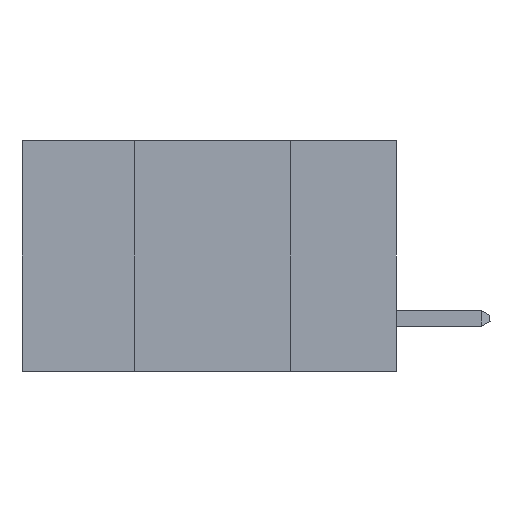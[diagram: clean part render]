
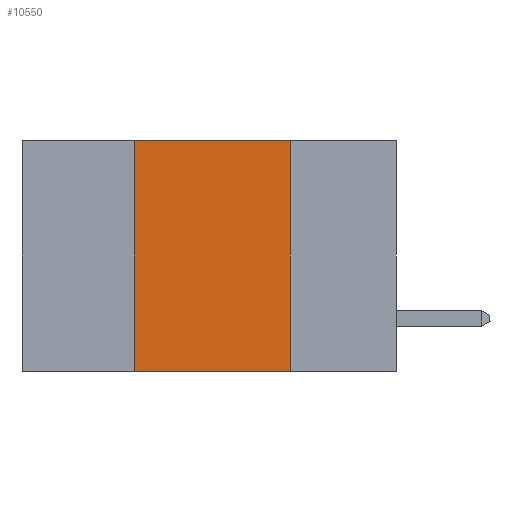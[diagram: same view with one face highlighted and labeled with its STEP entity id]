
A CAD part, left-side view. The second image highlights one B-rep face of the part: STEP entity #10550.
In plain terms, the highlighted planar face has unit normal (-1, 0, 0).
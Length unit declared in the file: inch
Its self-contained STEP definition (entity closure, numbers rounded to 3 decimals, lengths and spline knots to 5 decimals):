
#1699 = CARTESIAN_POINT ( 'NONE',  ( 0., 0.17, 0. ) ) ;
#2723 = DIRECTION ( 'NONE',  ( 0., 0., 1. ) ) ;
#2768 = CARTESIAN_POINT ( 'NONE',  ( 0., 0.17, 0. ) ) ;
#3005 = VERTEX_POINT ( 'NONE', #1699 ) ;
#3600 = EDGE_CURVE ( 'NONE', #3005, #13760, #9320, .T. ) ;
#3969 = CARTESIAN_POINT ( 'NONE',  ( 0., 0.6, -0.37 ) ) ;
#4650 = VERTEX_POINT ( 'NONE', #13246 ) ;
#6016 = VERTEX_POINT ( 'NONE', #13065 ) ;
#6227 = CARTESIAN_POINT ( 'NONE',  ( 0., 0.42, 0. ) ) ;
#6382 = ORIENTED_EDGE ( 'NONE', *, *, #3600, .F. ) ;
#6568 = VECTOR ( 'NONE', #2723, 39.37008 ) ;
#6905 = VECTOR ( 'NONE', #17287, 39.37008 ) ;
#7635 = AXIS2_PLACEMENT_3D ( 'NONE', #21035, #19313, #11101 ) ;
#7870 = EDGE_CURVE ( 'NONE', #4650, #3005, #17829, .T. ) ;
#8924 = CARTESIAN_POINT ( 'NONE',  ( 0., 0.6, 0. ) ) ;
#8963 = ORIENTED_EDGE ( 'NONE', *, *, #17254, .T. ) ;
#9320 = LINE ( 'NONE', #2768, #18553 ) ;
#10550 = ADVANCED_FACE ( 'NONE', ( #16448 ), #17581, .F. ) ;
#11101 = DIRECTION ( 'NONE',  ( 0., 0., -1. ) ) ;
#11475 = LINE ( 'NONE', #6227, #6568 ) ;
#11549 = EDGE_LOOP ( 'NONE', ( #6382, #18554, #17080, #8963 ) ) ;
#13065 = CARTESIAN_POINT ( 'NONE',  ( 0., 0.42, -0.37 ) ) ;
#13144 = VECTOR ( 'NONE', #17275, 39.37008 ) ;
#13246 = CARTESIAN_POINT ( 'NONE',  ( 0., 0.42, 0. ) ) ;
#13629 = LINE ( 'NONE', #3969, #6905 ) ;
#13760 = VERTEX_POINT ( 'NONE', #17978 ) ;
#15643 = EDGE_CURVE ( 'NONE', #6016, #4650, #11475, .T. ) ;
#16448 = FACE_OUTER_BOUND ( 'NONE', #11549, .T. ) ;
#17080 = ORIENTED_EDGE ( 'NONE', *, *, #15643, .F. ) ;
#17254 = EDGE_CURVE ( 'NONE', #6016, #13760, #13629, .T. ) ;
#17275 = DIRECTION ( 'NONE',  ( 0., -1., 0. ) ) ;
#17287 = DIRECTION ( 'NONE',  ( 0., -1., 0. ) ) ;
#17581 = PLANE ( 'NONE',  #7635 ) ;
#17829 = LINE ( 'NONE', #8924, #13144 ) ;
#17978 = CARTESIAN_POINT ( 'NONE',  ( 0., 0.17, -0.37 ) ) ;
#18553 = VECTOR ( 'NONE', #19533, 39.37008 ) ;
#18554 = ORIENTED_EDGE ( 'NONE', *, *, #7870, .F. ) ;
#19313 = DIRECTION ( 'NONE',  ( 1., 0., 0. ) ) ;
#19533 = DIRECTION ( 'NONE',  ( 0., 0., -1. ) ) ;
#21035 = CARTESIAN_POINT ( 'NONE',  ( 0., 0.6, 0. ) ) ;
